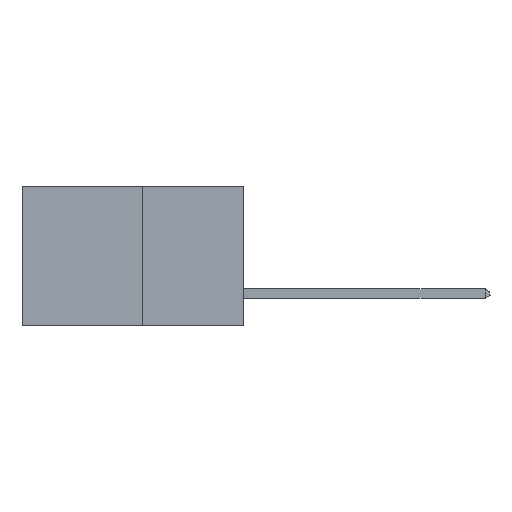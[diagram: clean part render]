
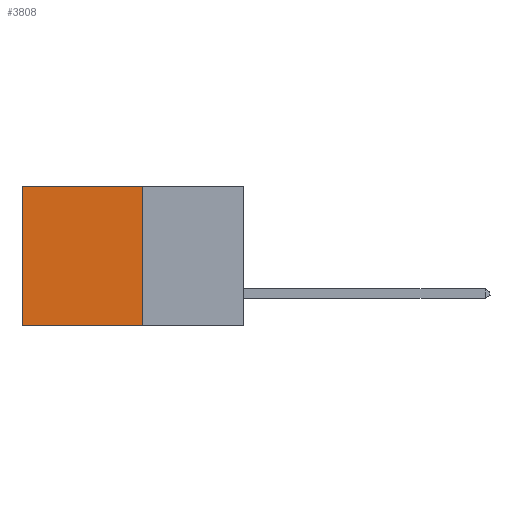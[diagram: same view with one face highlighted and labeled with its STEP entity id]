
A CAD part, left-side view. The second image highlights one B-rep face of the part: STEP entity #3808.
In plain terms, the highlighted planar face has unit normal (-1, 0, 0).
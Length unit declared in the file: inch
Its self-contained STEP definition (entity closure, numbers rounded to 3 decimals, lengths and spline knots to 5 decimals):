
#410 = CARTESIAN_POINT ( 'NONE',  ( 0.277, 0.27, -0.37 ) ) ;
#976 = DIRECTION ( 'NONE',  ( 0., 1., 0. ) ) ;
#1679 = CARTESIAN_POINT ( 'NONE',  ( 0.277, 0.27, 0. ) ) ;
#2110 = CARTESIAN_POINT ( 'NONE',  ( 0.277, 0.59, -0.37 ) ) ;
#3808 = ADVANCED_FACE ( 'NONE', ( #17770 ), #22347, .F. ) ;
#4164 = VECTOR ( 'NONE', #11884, 39.37008 ) ;
#4327 = LINE ( 'NONE', #1679, #24683 ) ;
#4330 = DIRECTION ( 'NONE',  ( 0., 1., 0. ) ) ;
#4760 = AXIS2_PLACEMENT_3D ( 'NONE', #24571, #24205, #23646 ) ;
#5973 = EDGE_CURVE ( 'NONE', #15571, #24126, #25938, .T. ) ;
#7427 = ORIENTED_EDGE ( 'NONE', *, *, #27968, .T. ) ;
#8759 = EDGE_CURVE ( 'NONE', #23198, #27713, #4327, .T. ) ;
#9305 = CARTESIAN_POINT ( 'NONE',  ( 0.277, 0.27, -0.37 ) ) ;
#9637 = ORIENTED_EDGE ( 'NONE', *, *, #10848, .F. ) ;
#10848 = EDGE_CURVE ( 'NONE', #23198, #15571, #24530, .T. ) ;
#11000 = CARTESIAN_POINT ( 'NONE',  ( 0.277, 0.59, -0.37 ) ) ;
#11884 = DIRECTION ( 'NONE',  ( 0., 0., -1. ) ) ;
#13576 = ORIENTED_EDGE ( 'NONE', *, *, #8759, .T. ) ;
#15571 = VERTEX_POINT ( 'NONE', #23970 ) ;
#16939 = ORIENTED_EDGE ( 'NONE', *, *, #5973, .F. ) ;
#17770 = FACE_OUTER_BOUND ( 'NONE', #31092, .T. ) ;
#22347 = PLANE ( 'NONE',  #4760 ) ;
#23198 = VERTEX_POINT ( 'NONE', #24538 ) ;
#23646 = DIRECTION ( 'NONE',  ( 0., 0., -1. ) ) ;
#23970 = CARTESIAN_POINT ( 'NONE',  ( 0.277, 0.27, -0.37 ) ) ;
#24126 = VERTEX_POINT ( 'NONE', #11000 ) ;
#24205 = DIRECTION ( 'NONE',  ( 1., 0., 0. ) ) ;
#24530 = LINE ( 'NONE', #9305, #4164 ) ;
#24538 = CARTESIAN_POINT ( 'NONE',  ( 0.277, 0.27, 0. ) ) ;
#24571 = CARTESIAN_POINT ( 'NONE',  ( 0.277, 0.27, -0.37 ) ) ;
#24683 = VECTOR ( 'NONE', #4330, 39.37008 ) ;
#24923 = VECTOR ( 'NONE', #32633, 39.37008 ) ;
#25148 = VECTOR ( 'NONE', #976, 39.37008 ) ;
#25938 = LINE ( 'NONE', #410, #25148 ) ;
#27713 = VERTEX_POINT ( 'NONE', #29331 ) ;
#27968 = EDGE_CURVE ( 'NONE', #27713, #24126, #31537, .T. ) ;
#29331 = CARTESIAN_POINT ( 'NONE',  ( 0.277, 0.59, 0. ) ) ;
#31092 = EDGE_LOOP ( 'NONE', ( #7427, #16939, #9637, #13576 ) ) ;
#31537 = LINE ( 'NONE', #2110, #24923 ) ;
#32633 = DIRECTION ( 'NONE',  ( 0., 0., -1. ) ) ;
